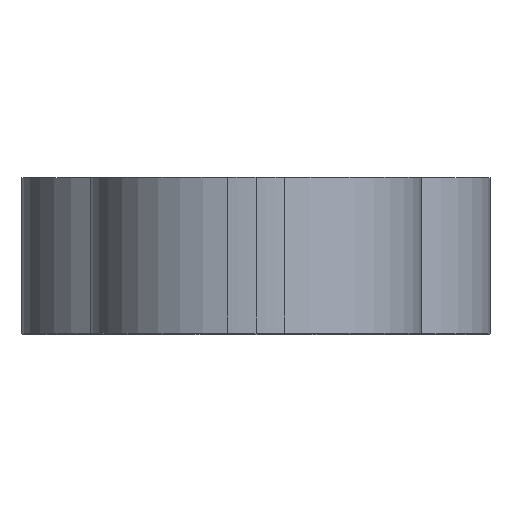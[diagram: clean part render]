
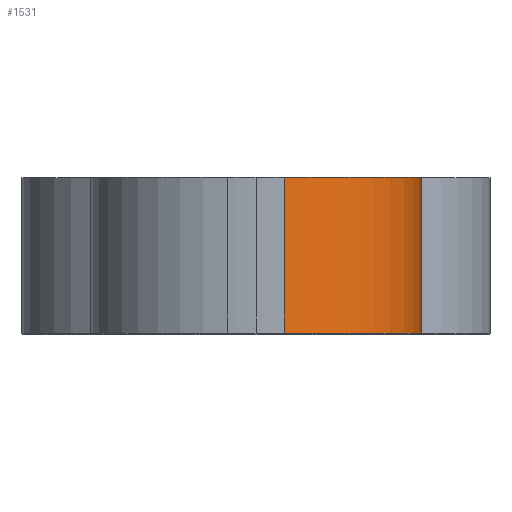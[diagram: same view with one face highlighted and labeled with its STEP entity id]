
A CAD part, top view. The second image highlights one B-rep face of the part: STEP entity #1531.
In plain terms, the highlighted cylindrical face has radius 5 mm (diameter 10 mm), a partial arc.
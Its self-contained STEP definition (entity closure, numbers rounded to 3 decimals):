
#3 = AXIS2_PLACEMENT_3D ( 'NONE', #454, #1019, #184 ) ;
#44 = CARTESIAN_POINT ( 'NONE',  ( 0.91, -2.5, 14.945 ) ) ;
#150 = AXIS2_PLACEMENT_3D ( 'NONE', #912, #364, #1294 ) ;
#184 = DIRECTION ( 'NONE',  ( 1., 0., 0. ) ) ;
#279 = VECTOR ( 'NONE', #1106, 1000. ) ;
#304 = LINE ( 'NONE', #1490, #279 ) ;
#311 = AXIS2_PLACEMENT_3D ( 'NONE', #1242, #1240, #1232 ) ;
#325 = VERTEX_POINT ( 'NONE', #383 ) ;
#364 = DIRECTION ( 'NONE',  ( 0., -1., 0. ) ) ;
#383 = CARTESIAN_POINT ( 'NONE',  ( 5.303, -2.5, 9.982 ) ) ;
#412 = EDGE_LOOP ( 'NONE', ( #1453, #1730, #657, #675 ) ) ;
#416 = CYLINDRICAL_SURFACE ( 'NONE', #3, 5. ) ;
#454 = CARTESIAN_POINT ( 'NONE',  ( 0.303, 0., 9.982 ) ) ;
#480 = FACE_OUTER_BOUND ( 'NONE', #412, .T. ) ;
#490 = CARTESIAN_POINT ( 'NONE',  ( 5.303, 2.5, 9.982 ) ) ;
#509 = EDGE_CURVE ( 'NONE', #1285, #325, #1405, .T. ) ;
#554 = EDGE_CURVE ( 'NONE', #1220, #1285, #1343, .T. ) ;
#654 = CIRCLE ( 'NONE', #150, 5. ) ;
#657 = ORIENTED_EDGE ( 'NONE', *, *, #554, .F. ) ;
#675 = ORIENTED_EDGE ( 'NONE', *, *, #1639, .F. ) ;
#912 = CARTESIAN_POINT ( 'NONE',  ( 0.303, -2.5, 9.982 ) ) ;
#1019 = DIRECTION ( 'NONE',  ( 0., -1., 0. ) ) ;
#1106 = DIRECTION ( 'NONE',  ( 0., 1., 0. ) ) ;
#1147 = VERTEX_POINT ( 'NONE', #44 ) ;
#1220 = VERTEX_POINT ( 'NONE', #1555 ) ;
#1232 = DIRECTION ( 'NONE',  ( 0., 0., -1. ) ) ;
#1240 = DIRECTION ( 'NONE',  ( 0., 1., 0. ) ) ;
#1242 = CARTESIAN_POINT ( 'NONE',  ( 0.303, 2.5, 9.982 ) ) ;
#1276 = EDGE_CURVE ( 'NONE', #325, #1147, #654, .T. ) ;
#1285 = VERTEX_POINT ( 'NONE', #490 ) ;
#1294 = DIRECTION ( 'NONE',  ( 0., 0., 1. ) ) ;
#1343 = CIRCLE ( 'NONE', #311, 5. ) ;
#1369 = DIRECTION ( 'NONE',  ( 0., -1., 0. ) ) ;
#1395 = VECTOR ( 'NONE', #1369, 1000. ) ;
#1405 = LINE ( 'NONE', #1410, #1395 ) ;
#1410 = CARTESIAN_POINT ( 'NONE',  ( 5.303, -2.5, 9.982 ) ) ;
#1453 = ORIENTED_EDGE ( 'NONE', *, *, #1276, .F. ) ;
#1490 = CARTESIAN_POINT ( 'NONE',  ( 0.91, 0., 14.945 ) ) ;
#1531 = ADVANCED_FACE ( 'NONE', ( #480 ), #416, .T. ) ;
#1555 = CARTESIAN_POINT ( 'NONE',  ( 0.91, 2.5, 14.945 ) ) ;
#1639 = EDGE_CURVE ( 'NONE', #1147, #1220, #304, .T. ) ;
#1730 = ORIENTED_EDGE ( 'NONE', *, *, #509, .F. ) ;
